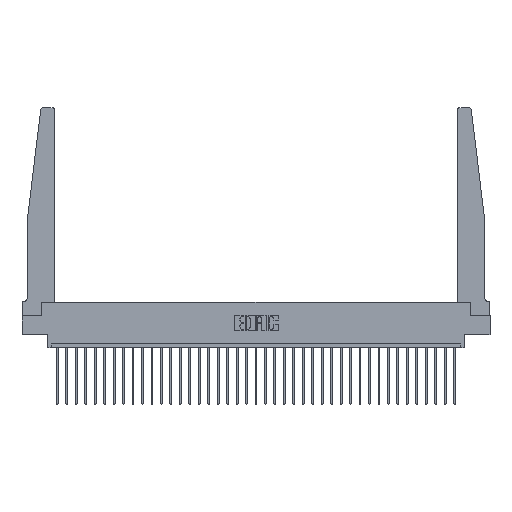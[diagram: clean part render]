
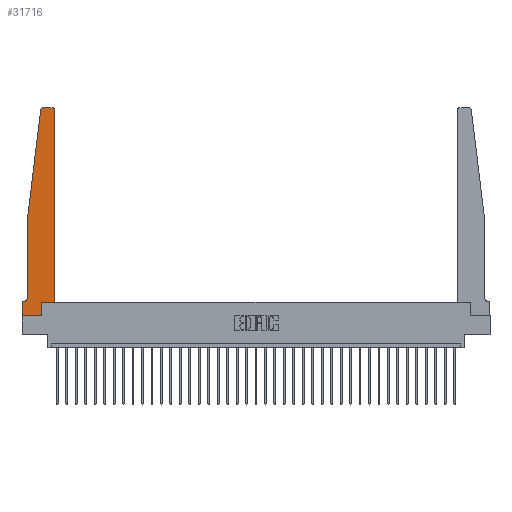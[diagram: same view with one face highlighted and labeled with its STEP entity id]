
A CAD part, top view. The second image highlights one B-rep face of the part: STEP entity #31716.
In plain terms, the highlighted planar face has unit normal (0, 0, 1).
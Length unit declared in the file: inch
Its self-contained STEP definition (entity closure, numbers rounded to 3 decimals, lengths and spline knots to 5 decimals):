
#29 = EDGE_CURVE ( 'NONE', #27583, #26187, #12846, .T. ) ;
#944 = ORIENTED_EDGE ( 'NONE', *, *, #29, .T. ) ;
#964 = VERTEX_POINT ( 'NONE', #22581 ) ;
#1205 = VERTEX_POINT ( 'NONE', #17664 ) ;
#1612 = CARTESIAN_POINT ( 'NONE',  ( 0.27653, 2.72, 0.37 ) ) ;
#1615 = DIRECTION ( 'NONE',  ( 1., 0., 0. ) ) ;
#3954 = DIRECTION ( 'NONE',  ( 1., 0., 0. ) ) ;
#4074 = VECTOR ( 'NONE', #12179, 39.37008 ) ;
#4344 = DIRECTION ( 'NONE',  ( 0., 0., 1. ) ) ;
#4405 = VECTOR ( 'NONE', #5990, 39.37008 ) ;
#4977 = LINE ( 'NONE', #22051, #12885 ) ;
#5855 = VECTOR ( 'NONE', #8455, 39.37008 ) ;
#5948 = VERTEX_POINT ( 'NONE', #25036 ) ;
#5990 = DIRECTION ( 'NONE',  ( 0., -1., 0. ) ) ;
#6008 = EDGE_CURVE ( 'NONE', #30186, #964, #17724, .T. ) ;
#6402 = CARTESIAN_POINT ( 'NONE',  ( 0.425, 0.18, 0.37 ) ) ;
#6704 = VERTEX_POINT ( 'NONE', #18299 ) ;
#7027 = CARTESIAN_POINT ( 'NONE',  ( 0.25, 2.75, 0.37 ) ) ;
#7350 = LINE ( 'NONE', #7027, #4074 ) ;
#7664 = EDGE_CURVE ( 'NONE', #24489, #1205, #21423, .T. ) ;
#7909 = LINE ( 'NONE', #10794, #19994 ) ;
#8285 = CARTESIAN_POINT ( 'NONE',  ( 0.2605, 0., 0.37 ) ) ;
#8351 = ORIENTED_EDGE ( 'NONE', *, *, #14466, .T. ) ;
#8455 = DIRECTION ( 'NONE',  ( 0., -1., 0. ) ) ;
#8534 = AXIS2_PLACEMENT_3D ( 'NONE', #1612, #21116, #11440 ) ;
#8560 = VERTEX_POINT ( 'NONE', #19840 ) ;
#9224 = VECTOR ( 'NONE', #21038, 39.37008 ) ;
#10381 = LINE ( 'NONE', #20222, #5855 ) ;
#10457 = ORIENTED_EDGE ( 'NONE', *, *, #21064, .T. ) ;
#10794 = CARTESIAN_POINT ( 'NONE',  ( 0.065, 0.1875, 0.37 ) ) ;
#11134 = CARTESIAN_POINT ( 'NONE',  ( 0.065, 1.25, 0.37 ) ) ;
#11440 = DIRECTION ( 'NONE',  ( 1., 0., 0. ) ) ;
#12179 = DIRECTION ( 'NONE',  ( -1., 0., 0. ) ) ;
#12274 = EDGE_CURVE ( 'NONE', #13677, #6704, #17433, .T. ) ;
#12739 = DIRECTION ( 'NONE',  ( -1., 0., 0. ) ) ;
#12802 = EDGE_CURVE ( 'NONE', #5948, #17714, #7909, .T. ) ;
#12846 = LINE ( 'NONE', #13633, #9224 ) ;
#12885 = VECTOR ( 'NONE', #21896, 39.37008 ) ;
#12908 = CARTESIAN_POINT ( 'NONE',  ( 0.395, 2.72, 0.37 ) ) ;
#13483 = CARTESIAN_POINT ( 'NONE',  ( 0., 0., 0.37 ) ) ;
#13633 = CARTESIAN_POINT ( 'NONE',  ( 0.425, 0.18, 0.37 ) ) ;
#13677 = VERTEX_POINT ( 'NONE', #8285 ) ;
#13866 = CARTESIAN_POINT ( 'NONE',  ( 0., 0.1875, 0.37 ) ) ;
#14466 = EDGE_CURVE ( 'NONE', #964, #24489, #4977, .T. ) ;
#14731 = ORIENTED_EDGE ( 'NONE', *, *, #12802, .T. ) ;
#15309 = EDGE_CURVE ( 'NONE', #30692, #13677, #26041, .T. ) ;
#15476 = ORIENTED_EDGE ( 'NONE', *, *, #25543, .T. ) ;
#15887 = CARTESIAN_POINT ( 'NONE',  ( 0.015, 0.2375, 0.37 ) ) ;
#17126 = AXIS2_PLACEMENT_3D ( 'NONE', #15887, #23152, #18312 ) ;
#17433 = LINE ( 'NONE', #26820, #20507 ) ;
#17664 = CARTESIAN_POINT ( 'NONE',  ( 0.065, 0.2375, 0.37 ) ) ;
#17714 = VERTEX_POINT ( 'NONE', #26442 ) ;
#17724 = CIRCLE ( 'NONE', #8534, 0.03 ) ;
#18299 = CARTESIAN_POINT ( 'NONE',  ( 0.2605, 0.18, 0.37 ) ) ;
#18312 = DIRECTION ( 'NONE',  ( -1., 0., 0. ) ) ;
#18317 = VECTOR ( 'NONE', #24568, 39.37008 ) ;
#18398 = EDGE_CURVE ( 'NONE', #1205, #5948, #24883, .T. ) ;
#19840 = CARTESIAN_POINT ( 'NONE',  ( 0.395, 2.75, 0.37 ) ) ;
#19993 = ORIENTED_EDGE ( 'NONE', *, *, #12274, .T. ) ;
#19994 = VECTOR ( 'NONE', #12739, 39.37008 ) ;
#20222 = CARTESIAN_POINT ( 'NONE',  ( 0., 0., 0.37 ) ) ;
#20257 = EDGE_CURVE ( 'NONE', #17714, #30692, #10381, .T. ) ;
#20507 = VECTOR ( 'NONE', #22121, 39.37008 ) ;
#21007 = CARTESIAN_POINT ( 'NONE',  ( 0.425, 2.72, 0.37 ) ) ;
#21038 = DIRECTION ( 'NONE',  ( 0., 1., 0. ) ) ;
#21064 = EDGE_CURVE ( 'NONE', #26187, #8560, #26956, .T. ) ;
#21116 = DIRECTION ( 'NONE',  ( 0., 0., 1. ) ) ;
#21423 = LINE ( 'NONE', #11134, #4405 ) ;
#21646 = VECTOR ( 'NONE', #3954, 39.37008 ) ;
#21896 = DIRECTION ( 'NONE',  ( -0.122, -0.992, 0. ) ) ;
#22051 = CARTESIAN_POINT ( 'NONE',  ( 0.065, 1.25, 0.37 ) ) ;
#22121 = DIRECTION ( 'NONE',  ( 0., 1., 0. ) ) ;
#22581 = CARTESIAN_POINT ( 'NONE',  ( 0.24675, 2.72367, 0.37 ) ) ;
#23152 = DIRECTION ( 'NONE',  ( 0., 0., -1. ) ) ;
#23372 = FACE_OUTER_BOUND ( 'NONE', #24495, .T. ) ;
#24088 = CARTESIAN_POINT ( 'NONE',  ( 0.425, 0.18, 0.37 ) ) ;
#24197 = CARTESIAN_POINT ( 'NONE',  ( 0.27653, 2.75, 0.37 ) ) ;
#24489 = VERTEX_POINT ( 'NONE', #29090 ) ;
#24495 = EDGE_LOOP ( 'NONE', ( #25053, #30736, #8351, #24675, #30635, #14731, #31595, #31885, #19993, #15476, #944, #10457 ) ) ;
#24568 = DIRECTION ( 'NONE',  ( 1., 0., 0. ) ) ;
#24675 = ORIENTED_EDGE ( 'NONE', *, *, #7664, .T. ) ;
#24743 = LINE ( 'NONE', #24088, #18317 ) ;
#24883 = CIRCLE ( 'NONE', #17126, 0.05 ) ;
#25036 = CARTESIAN_POINT ( 'NONE',  ( 0.015, 0.1875, 0.37 ) ) ;
#25053 = ORIENTED_EDGE ( 'NONE', *, *, #29040, .T. ) ;
#25147 = DIRECTION ( 'NONE',  ( 0., 0., 1. ) ) ;
#25227 = AXIS2_PLACEMENT_3D ( 'NONE', #13866, #4344, #1615 ) ;
#25543 = EDGE_CURVE ( 'NONE', #6704, #27583, #24743, .T. ) ;
#25881 = CARTESIAN_POINT ( 'NONE',  ( 0., 0., 0.37 ) ) ;
#25962 = PLANE ( 'NONE',  #25227 ) ;
#26041 = LINE ( 'NONE', #13483, #21646 ) ;
#26187 = VERTEX_POINT ( 'NONE', #21007 ) ;
#26442 = CARTESIAN_POINT ( 'NONE',  ( 0., 0.1875, 0.37 ) ) ;
#26820 = CARTESIAN_POINT ( 'NONE',  ( 0.2605, 0.18, 0.37 ) ) ;
#26956 = CIRCLE ( 'NONE', #31094, 0.03 ) ;
#27583 = VERTEX_POINT ( 'NONE', #6402 ) ;
#27911 = DIRECTION ( 'NONE',  ( 1., 0., 0. ) ) ;
#29040 = EDGE_CURVE ( 'NONE', #8560, #30186, #7350, .T. ) ;
#29090 = CARTESIAN_POINT ( 'NONE',  ( 0.065, 1.25, 0.37 ) ) ;
#30186 = VERTEX_POINT ( 'NONE', #24197 ) ;
#30635 = ORIENTED_EDGE ( 'NONE', *, *, #18398, .T. ) ;
#30692 = VERTEX_POINT ( 'NONE', #25881 ) ;
#30736 = ORIENTED_EDGE ( 'NONE', *, *, #6008, .T. ) ;
#31094 = AXIS2_PLACEMENT_3D ( 'NONE', #12908, #25147, #27911 ) ;
#31595 = ORIENTED_EDGE ( 'NONE', *, *, #20257, .T. ) ;
#31716 = ADVANCED_FACE ( 'NONE', ( #23372 ), #25962, .T. ) ;
#31885 = ORIENTED_EDGE ( 'NONE', *, *, #15309, .T. ) ;
